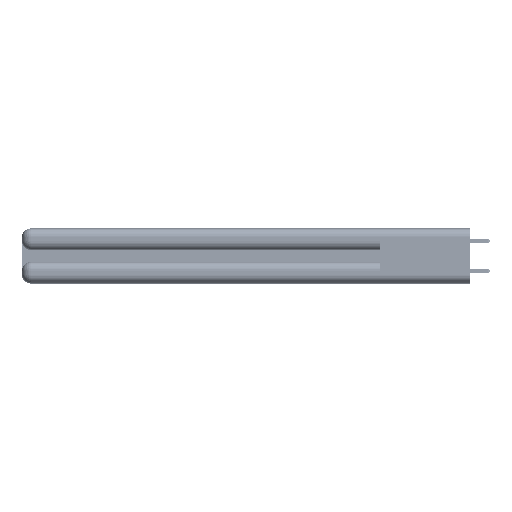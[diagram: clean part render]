
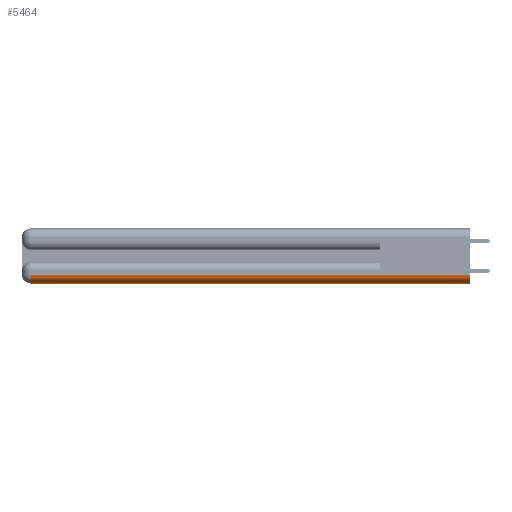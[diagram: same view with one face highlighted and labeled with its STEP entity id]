
A CAD part, left-side view. The second image highlights one B-rep face of the part: STEP entity #5464.
In plain terms, the highlighted cylindrical face has radius 1.524 mm (diameter 3.048 mm), a partial arc.
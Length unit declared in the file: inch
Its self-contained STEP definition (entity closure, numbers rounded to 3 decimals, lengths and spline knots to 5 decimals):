
#2090 = CARTESIAN_POINT ( 'NONE',  ( 0.06, 0., 0. ) ) ;
#2844 = CIRCLE ( 'NONE', #24842, 0.06 ) ;
#3113 = EDGE_LOOP ( 'NONE', ( #46102, #12892, #52996, #32658 ) ) ;
#3665 = CIRCLE ( 'NONE', #13698, 0.06 ) ;
#5464 = ADVANCED_FACE ( 'NONE', ( #43531 ), #51713, .T. ) ;
#7598 = VERTEX_POINT ( 'NONE', #34024 ) ;
#8089 = DIRECTION ( 'NONE',  ( 0., 0., 1. ) ) ;
#8124 = CARTESIAN_POINT ( 'NONE',  ( 0.06, 0., 0.06 ) ) ;
#8136 = DIRECTION ( 'NONE',  ( 0., 1., 0. ) ) ;
#8317 = CARTESIAN_POINT ( 'NONE',  ( 0.06, 3., 0. ) ) ;
#11989 = LINE ( 'NONE', #8317, #22910 ) ;
#12892 = ORIENTED_EDGE ( 'NONE', *, *, #48606, .F. ) ;
#13318 = DIRECTION ( 'NONE',  ( 0., -1., 0. ) ) ;
#13698 = AXIS2_PLACEMENT_3D ( 'NONE', #14284, #18090, #27088 ) ;
#14284 = CARTESIAN_POINT ( 'NONE',  ( 0.06, 2.94, 0.06 ) ) ;
#18090 = DIRECTION ( 'NONE',  ( 0., 1., 0. ) ) ;
#19142 = AXIS2_PLACEMENT_3D ( 'NONE', #8124, #47750, #47190 ) ;
#22349 = VERTEX_POINT ( 'NONE', #2090 ) ;
#22910 = VECTOR ( 'NONE', #8136, 39.37008 ) ;
#24842 = AXIS2_PLACEMENT_3D ( 'NONE', #25447, #29799, #8089 ) ;
#25447 = CARTESIAN_POINT ( 'NONE',  ( 0.06, 0., 0.06 ) ) ;
#27088 = DIRECTION ( 'NONE',  ( 0., 0., 1. ) ) ;
#29702 = EDGE_CURVE ( 'NONE', #7598, #50689, #3665, .T. ) ;
#29799 = DIRECTION ( 'NONE',  ( 0., -1., 0. ) ) ;
#32658 = ORIENTED_EDGE ( 'NONE', *, *, #35076, .F. ) ;
#34024 = CARTESIAN_POINT ( 'NONE',  ( 0.06, 2.94, 0. ) ) ;
#35076 = EDGE_CURVE ( 'NONE', #22349, #7598, #11989, .T. ) ;
#40302 = EDGE_CURVE ( 'NONE', #56374, #22349, #2844, .T. ) ;
#43531 = FACE_OUTER_BOUND ( 'NONE', #3113, .T. ) ;
#44024 = VECTOR ( 'NONE', #13318, 39.37008 ) ;
#46102 = ORIENTED_EDGE ( 'NONE', *, *, #40302, .F. ) ;
#46112 = LINE ( 'NONE', #47836, #44024 ) ;
#47190 = DIRECTION ( 'NONE',  ( 0., 0., 1. ) ) ;
#47750 = DIRECTION ( 'NONE',  ( 0., 1., 0. ) ) ;
#47836 = CARTESIAN_POINT ( 'NONE',  ( 0., 0., 0.06 ) ) ;
#48606 = EDGE_CURVE ( 'NONE', #50689, #56374, #46112, .T. ) ;
#50689 = VERTEX_POINT ( 'NONE', #52307 ) ;
#51713 = CYLINDRICAL_SURFACE ( 'NONE', #19142, 0.06 ) ;
#52307 = CARTESIAN_POINT ( 'NONE',  ( 0., 2.94, 0.06 ) ) ;
#52507 = CARTESIAN_POINT ( 'NONE',  ( 0., 0., 0.06 ) ) ;
#52996 = ORIENTED_EDGE ( 'NONE', *, *, #29702, .F. ) ;
#56374 = VERTEX_POINT ( 'NONE', #52507 ) ;
